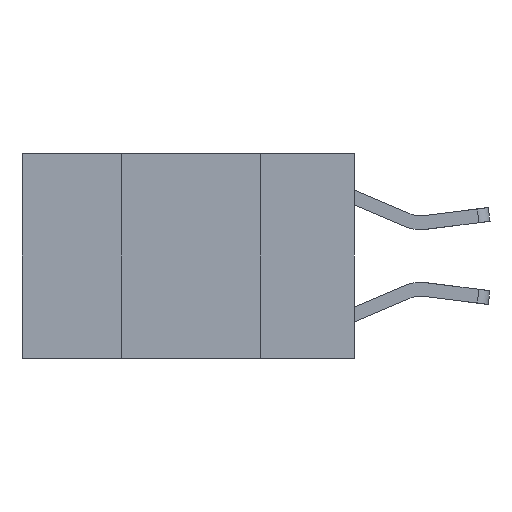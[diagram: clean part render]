
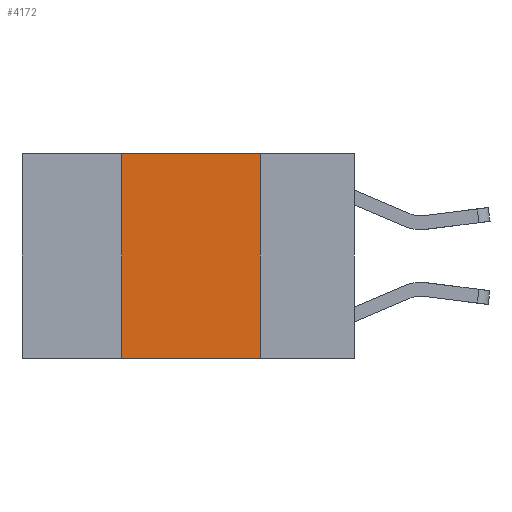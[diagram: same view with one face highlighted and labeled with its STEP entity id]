
A CAD part, left-side view. The second image highlights one B-rep face of the part: STEP entity #4172.
In plain terms, the highlighted planar face has unit normal (-1, 0, 0).
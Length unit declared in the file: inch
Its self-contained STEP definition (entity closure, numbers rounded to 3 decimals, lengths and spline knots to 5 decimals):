
#241 = EDGE_LOOP ( 'NONE', ( #6157, #8105, #828, #8787 ) ) ;
#283 = DIRECTION ( 'NONE',  ( 1., 0., 0. ) ) ;
#459 = DIRECTION ( 'NONE',  ( 0., -1., 0. ) ) ;
#828 = ORIENTED_EDGE ( 'NONE', *, *, #3761, .F. ) ;
#871 = LINE ( 'NONE', #3719, #5185 ) ;
#962 = DIRECTION ( 'NONE',  ( 0., -1., 0. ) ) ;
#1457 = AXIS2_PLACEMENT_3D ( 'NONE', #7810, #283, #2237 ) ;
#1502 = CARTESIAN_POINT ( 'NONE',  ( 0., 0.17, -0.37 ) ) ;
#1767 = VERTEX_POINT ( 'NONE', #1502 ) ;
#2237 = DIRECTION ( 'NONE',  ( 0., 0., -1. ) ) ;
#2311 = VECTOR ( 'NONE', #459, 39.37008 ) ;
#2419 = DIRECTION ( 'NONE',  ( 0., 0., 1. ) ) ;
#3283 = EDGE_CURVE ( 'NONE', #7626, #5726, #3778, .T. ) ;
#3333 = VECTOR ( 'NONE', #6580, 39.37008 ) ;
#3719 = CARTESIAN_POINT ( 'NONE',  ( 0., 0.42, 0. ) ) ;
#3761 = EDGE_CURVE ( 'NONE', #4579, #7626, #871, .T. ) ;
#3778 = LINE ( 'NONE', #5844, #2311 ) ;
#4172 = ADVANCED_FACE ( 'NONE', ( #8347 ), #7004, .F. ) ;
#4200 = CARTESIAN_POINT ( 'NONE',  ( 0., 0.42, 0. ) ) ;
#4579 = VERTEX_POINT ( 'NONE', #8232 ) ;
#4631 = LINE ( 'NONE', #6622, #3333 ) ;
#5185 = VECTOR ( 'NONE', #2419, 39.37008 ) ;
#5726 = VERTEX_POINT ( 'NONE', #8134 ) ;
#5798 = LINE ( 'NONE', #7055, #7046 ) ;
#5844 = CARTESIAN_POINT ( 'NONE',  ( 0., 0.6, 0. ) ) ;
#6157 = ORIENTED_EDGE ( 'NONE', *, *, #7143, .F. ) ;
#6506 = EDGE_CURVE ( 'NONE', #4579, #1767, #5798, .T. ) ;
#6580 = DIRECTION ( 'NONE',  ( 0., 0., -1. ) ) ;
#6622 = CARTESIAN_POINT ( 'NONE',  ( 0., 0.17, 0. ) ) ;
#7004 = PLANE ( 'NONE',  #1457 ) ;
#7046 = VECTOR ( 'NONE', #962, 39.37008 ) ;
#7055 = CARTESIAN_POINT ( 'NONE',  ( 0., 0.6, -0.37 ) ) ;
#7143 = EDGE_CURVE ( 'NONE', #5726, #1767, #4631, .T. ) ;
#7626 = VERTEX_POINT ( 'NONE', #4200 ) ;
#7810 = CARTESIAN_POINT ( 'NONE',  ( 0., 0.6, 0. ) ) ;
#8105 = ORIENTED_EDGE ( 'NONE', *, *, #3283, .F. ) ;
#8134 = CARTESIAN_POINT ( 'NONE',  ( 0., 0.17, 0. ) ) ;
#8232 = CARTESIAN_POINT ( 'NONE',  ( 0., 0.42, -0.37 ) ) ;
#8347 = FACE_OUTER_BOUND ( 'NONE', #241, .T. ) ;
#8787 = ORIENTED_EDGE ( 'NONE', *, *, #6506, .T. ) ;
